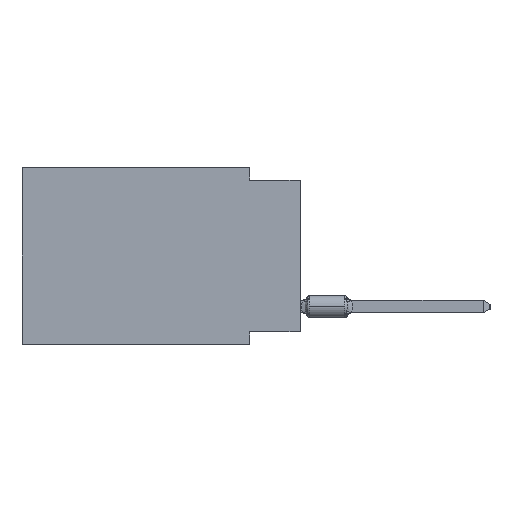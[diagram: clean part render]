
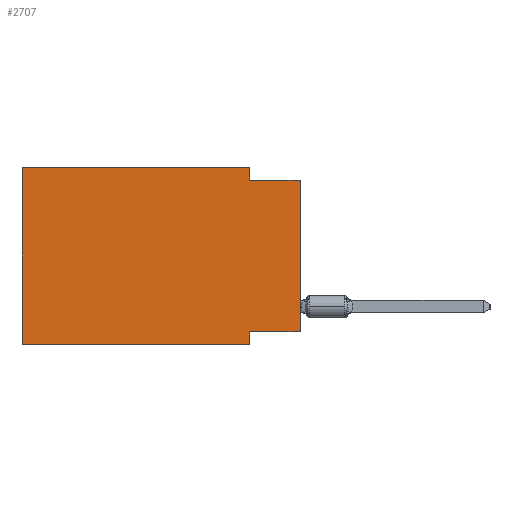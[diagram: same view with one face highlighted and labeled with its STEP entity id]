
A CAD part, left-side view. The second image highlights one B-rep face of the part: STEP entity #2707.
In plain terms, the highlighted planar face has unit normal (-1, 0, 0).
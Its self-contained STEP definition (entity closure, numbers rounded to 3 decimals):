
#10 = LINE ( 'NONE', #16747, #23096 ) ;
#1025 = VECTOR ( 'NONE', #30732, 1000. ) ;
#1058 = DIRECTION ( 'NONE',  ( 0., 0., 1. ) ) ;
#2432 = LINE ( 'NONE', #22443, #25118 ) ;
#2576 = VERTEX_POINT ( 'NONE', #7521 ) ;
#2697 = EDGE_CURVE ( 'NONE', #4704, #17738, #2432, .T. ) ;
#2707 = ADVANCED_FACE ( 'NONE', ( #16968 ), #30823, .F. ) ;
#3093 = DIRECTION ( 'NONE',  ( 0., -1., 0. ) ) ;
#4111 = DIRECTION ( 'NONE',  ( 0., 0., -1. ) ) ;
#4467 = VERTEX_POINT ( 'NONE', #11294 ) ;
#4704 = VERTEX_POINT ( 'NONE', #18731 ) ;
#6327 = DIRECTION ( 'NONE',  ( 0., -1., 0. ) ) ;
#6669 = EDGE_CURVE ( 'NONE', #8630, #21739, #32340, .T. ) ;
#7058 = EDGE_CURVE ( 'NONE', #2576, #17738, #20156, .T. ) ;
#7511 = VECTOR ( 'NONE', #4111, 1000. ) ;
#7521 = CARTESIAN_POINT ( 'NONE',  ( 0., 13.97, -8.89 ) ) ;
#7782 = VERTEX_POINT ( 'NONE', #28418 ) ;
#7807 = VECTOR ( 'NONE', #3093, 1000. ) ;
#8630 = VERTEX_POINT ( 'NONE', #14134 ) ;
#8729 = CARTESIAN_POINT ( 'NONE',  ( 0., 13.97, 0. ) ) ;
#8767 = DIRECTION ( 'NONE',  ( 0., 0., -1. ) ) ;
#8768 = VECTOR ( 'NONE', #1058, 1000. ) ;
#9179 = VERTEX_POINT ( 'NONE', #23493 ) ;
#9846 = EDGE_CURVE ( 'NONE', #9179, #4704, #19615, .T. ) ;
#11294 = CARTESIAN_POINT ( 'NONE',  ( 0., 0., -0.635 ) ) ;
#11920 = ORIENTED_EDGE ( 'NONE', *, *, #7058, .T. ) ;
#14082 = AXIS2_PLACEMENT_3D ( 'NONE', #19704, #27727, #28072 ) ;
#14134 = CARTESIAN_POINT ( 'NONE',  ( 0., 2.54, 0. ) ) ;
#15269 = ORIENTED_EDGE ( 'NONE', *, *, #9846, .F. ) ;
#15615 = ORIENTED_EDGE ( 'NONE', *, *, #34213, .F. ) ;
#16747 = CARTESIAN_POINT ( 'NONE',  ( 0., 13.97, 0. ) ) ;
#16968 = FACE_OUTER_BOUND ( 'NONE', #19905, .T. ) ;
#17051 = CARTESIAN_POINT ( 'NONE',  ( 0., 0., -8.255 ) ) ;
#17738 = VERTEX_POINT ( 'NONE', #20346 ) ;
#18481 = CARTESIAN_POINT ( 'NONE',  ( 0., 2.54, 0. ) ) ;
#18731 = CARTESIAN_POINT ( 'NONE',  ( 0., 2.54, -8.255 ) ) ;
#19280 = EDGE_CURVE ( 'NONE', #2576, #7782, #10, .T. ) ;
#19615 = LINE ( 'NONE', #17051, #1025 ) ;
#19704 = CARTESIAN_POINT ( 'NONE',  ( 0., 13.97, 0. ) ) ;
#19905 = EDGE_LOOP ( 'NONE', ( #31729, #35133, #30890, #15615, #35626, #11920, #22606, #15269 ) ) ;
#20156 = LINE ( 'NONE', #32979, #33710 ) ;
#20344 = LINE ( 'NONE', #31650, #24175 ) ;
#20346 = CARTESIAN_POINT ( 'NONE',  ( 0., 2.54, -8.89 ) ) ;
#21739 = VERTEX_POINT ( 'NONE', #29314 ) ;
#22252 = EDGE_CURVE ( 'NONE', #21739, #4467, #20344, .T. ) ;
#22443 = CARTESIAN_POINT ( 'NONE',  ( 0., 2.54, -8.89 ) ) ;
#22582 = LINE ( 'NONE', #8729, #7807 ) ;
#22606 = ORIENTED_EDGE ( 'NONE', *, *, #2697, .F. ) ;
#23096 = VECTOR ( 'NONE', #27862, 1000. ) ;
#23493 = CARTESIAN_POINT ( 'NONE',  ( 0., 0., -8.255 ) ) ;
#24175 = VECTOR ( 'NONE', #6327, 1000. ) ;
#25118 = VECTOR ( 'NONE', #8767, 1000. ) ;
#25990 = CARTESIAN_POINT ( 'NONE',  ( 0., 0., 0. ) ) ;
#26776 = EDGE_CURVE ( 'NONE', #9179, #4467, #28725, .T. ) ;
#27727 = DIRECTION ( 'NONE',  ( 1., 0., 0. ) ) ;
#27862 = DIRECTION ( 'NONE',  ( 0., 0., 1. ) ) ;
#28072 = DIRECTION ( 'NONE',  ( 0., 0., -1. ) ) ;
#28418 = CARTESIAN_POINT ( 'NONE',  ( 0., 13.97, 0. ) ) ;
#28725 = LINE ( 'NONE', #25990, #8768 ) ;
#29314 = CARTESIAN_POINT ( 'NONE',  ( 0., 2.54, -0.635 ) ) ;
#30732 = DIRECTION ( 'NONE',  ( 0., 1., 0. ) ) ;
#30823 = PLANE ( 'NONE',  #14082 ) ;
#30890 = ORIENTED_EDGE ( 'NONE', *, *, #6669, .F. ) ;
#31281 = DIRECTION ( 'NONE',  ( 0., -1., 0. ) ) ;
#31650 = CARTESIAN_POINT ( 'NONE',  ( 0., 0., -0.635 ) ) ;
#31729 = ORIENTED_EDGE ( 'NONE', *, *, #26776, .T. ) ;
#32340 = LINE ( 'NONE', #18481, #7511 ) ;
#32979 = CARTESIAN_POINT ( 'NONE',  ( 0., 13.97, -8.89 ) ) ;
#33710 = VECTOR ( 'NONE', #31281, 1000. ) ;
#34213 = EDGE_CURVE ( 'NONE', #7782, #8630, #22582, .T. ) ;
#35133 = ORIENTED_EDGE ( 'NONE', *, *, #22252, .F. ) ;
#35626 = ORIENTED_EDGE ( 'NONE', *, *, #19280, .F. ) ;
